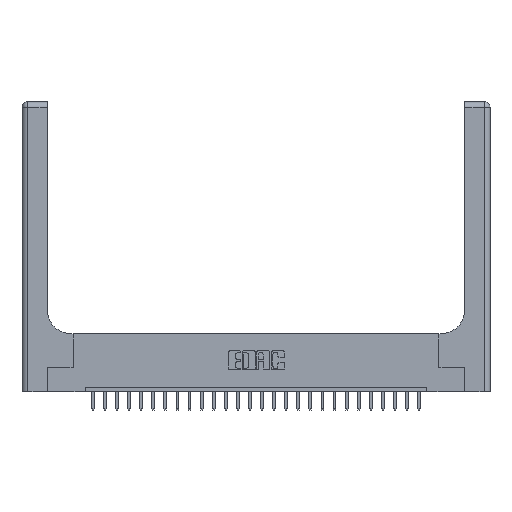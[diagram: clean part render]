
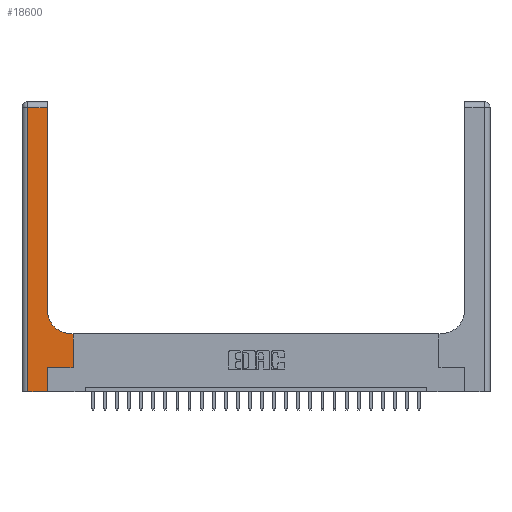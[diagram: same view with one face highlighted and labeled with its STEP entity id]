
A CAD part, top view. The second image highlights one B-rep face of the part: STEP entity #18600.
In plain terms, the highlighted planar face has unit normal (0, 0, 1).
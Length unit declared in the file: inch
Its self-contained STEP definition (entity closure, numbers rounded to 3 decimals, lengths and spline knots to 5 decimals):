
#73 = CARTESIAN_POINT ( 'NONE',  ( 0., 3., 0.37 ) ) ;
#515 = VERTEX_POINT ( 'NONE', #4664 ) ;
#550 = AXIS2_PLACEMENT_3D ( 'NONE', #73, #19193, #1833 ) ;
#741 = CARTESIAN_POINT ( 'NONE',  ( 0., 2.94, 0.37 ) ) ;
#776 = CARTESIAN_POINT ( 'NONE',  ( 0.06, 3., 0.37 ) ) ;
#839 = VECTOR ( 'NONE', #3467, 39.37008 ) ;
#1012 = VERTEX_POINT ( 'NONE', #14244 ) ;
#1243 = ORIENTED_EDGE ( 'NONE', *, *, #19330, .T. ) ;
#1570 = CARTESIAN_POINT ( 'NONE',  ( 0.528, 0.25, 0.37 ) ) ;
#1833 = DIRECTION ( 'NONE',  ( -1., 0., 0. ) ) ;
#2036 = EDGE_CURVE ( 'NONE', #1012, #13675, #19128, .T. ) ;
#2905 = DIRECTION ( 'NONE',  ( 0., -1., 0. ) ) ;
#3044 = DIRECTION ( 'NONE',  ( 0., 1., 0. ) ) ;
#3467 = DIRECTION ( 'NONE',  ( 0., 1., 0. ) ) ;
#3797 = DIRECTION ( 'NONE',  ( 1., 0., 0. ) ) ;
#3840 = ORIENTED_EDGE ( 'NONE', *, *, #20838, .T. ) ;
#3922 = CARTESIAN_POINT ( 'NONE',  ( 0.26, 0.6, 0.37 ) ) ;
#4664 = CARTESIAN_POINT ( 'NONE',  ( 0.06, 2.94, 0.37 ) ) ;
#4860 = VERTEX_POINT ( 'NONE', #6270 ) ;
#4895 = CARTESIAN_POINT ( 'NONE',  ( 0.265, 0., 0.37 ) ) ;
#5770 = DIRECTION ( 'NONE',  ( 0., 0., -1. ) ) ;
#5779 = VERTEX_POINT ( 'NONE', #9205 ) ;
#5790 = EDGE_LOOP ( 'NONE', ( #1243, #3840, #23263, #8727, #20140, #9080, #13010, #18107, #13633 ) ) ;
#6062 = CARTESIAN_POINT ( 'NONE',  ( 0.265, 0.25, 0.37 ) ) ;
#6270 = CARTESIAN_POINT ( 'NONE',  ( 0.06, 0., 0.37 ) ) ;
#7273 = VECTOR ( 'NONE', #23653, 39.37008 ) ;
#7275 = CARTESIAN_POINT ( 'NONE',  ( 0.528, 0.6, 0.37 ) ) ;
#7510 = VERTEX_POINT ( 'NONE', #7275 ) ;
#7710 = VECTOR ( 'NONE', #13552, 39.37008 ) ;
#8296 = CARTESIAN_POINT ( 'NONE',  ( 0.26, 2.94, 0.37 ) ) ;
#8441 = DIRECTION ( 'NONE',  ( -1., 0., 0. ) ) ;
#8727 = ORIENTED_EDGE ( 'NONE', *, *, #12777, .T. ) ;
#9080 = ORIENTED_EDGE ( 'NONE', *, *, #2036, .T. ) ;
#9205 = CARTESIAN_POINT ( 'NONE',  ( 0.26, 0.85, 0.37 ) ) ;
#9413 = FACE_OUTER_BOUND ( 'NONE', #5790, .T. ) ;
#9996 = CARTESIAN_POINT ( 'NONE',  ( 0.51, 0.6, 0.37 ) ) ;
#10021 = LINE ( 'NONE', #15847, #12925 ) ;
#10507 = LINE ( 'NONE', #14680, #18764 ) ;
#11520 = EDGE_CURVE ( 'NONE', #7510, #13034, #19633, .T. ) ;
#11776 = CARTESIAN_POINT ( 'NONE',  ( 0.528, 0.25, 0.37 ) ) ;
#11899 = LINE ( 'NONE', #11776, #7710 ) ;
#12273 = LINE ( 'NONE', #776, #13509 ) ;
#12777 = EDGE_CURVE ( 'NONE', #4860, #14941, #10021, .T. ) ;
#12925 = VECTOR ( 'NONE', #16975, 39.37008 ) ;
#13010 = ORIENTED_EDGE ( 'NONE', *, *, #14116, .T. ) ;
#13034 = VERTEX_POINT ( 'NONE', #9996 ) ;
#13509 = VECTOR ( 'NONE', #2905, 39.37008 ) ;
#13543 = VECTOR ( 'NONE', #8441, 39.37008 ) ;
#13552 = DIRECTION ( 'NONE',  ( 0., 1., 0. ) ) ;
#13611 = EDGE_CURVE ( 'NONE', #14941, #1012, #22964, .T. ) ;
#13633 = ORIENTED_EDGE ( 'NONE', *, *, #16988, .T. ) ;
#13675 = VERTEX_POINT ( 'NONE', #1570 ) ;
#14116 = EDGE_CURVE ( 'NONE', #13675, #7510, #11899, .T. ) ;
#14244 = CARTESIAN_POINT ( 'NONE',  ( 0.265, 0.25, 0.37 ) ) ;
#14680 = CARTESIAN_POINT ( 'NONE',  ( 0.26, 3., 0.37 ) ) ;
#14941 = VERTEX_POINT ( 'NONE', #4895 ) ;
#15847 = CARTESIAN_POINT ( 'NONE',  ( 0., 0., 0.37 ) ) ;
#16975 = DIRECTION ( 'NONE',  ( 1., 0., 0. ) ) ;
#16988 = EDGE_CURVE ( 'NONE', #13034, #5779, #17922, .T. ) ;
#17303 = DIRECTION ( 'NONE',  ( 1., 0., 0. ) ) ;
#17399 = PLANE ( 'NONE',  #550 ) ;
#17922 = CIRCLE ( 'NONE', #19168, 0.25 ) ;
#18107 = ORIENTED_EDGE ( 'NONE', *, *, #11520, .T. ) ;
#18186 = EDGE_CURVE ( 'NONE', #515, #4860, #12273, .T. ) ;
#18600 = ADVANCED_FACE ( 'NONE', ( #9413 ), #17399, .F. ) ;
#18764 = VECTOR ( 'NONE', #3044, 39.37008 ) ;
#19128 = LINE ( 'NONE', #6062, #22414 ) ;
#19168 = AXIS2_PLACEMENT_3D ( 'NONE', #20996, #5770, #17303 ) ;
#19193 = DIRECTION ( 'NONE',  ( 0., 0., -1. ) ) ;
#19330 = EDGE_CURVE ( 'NONE', #5779, #22185, #10507, .T. ) ;
#19633 = LINE ( 'NONE', #3922, #7273 ) ;
#20140 = ORIENTED_EDGE ( 'NONE', *, *, #13611, .T. ) ;
#20705 = CARTESIAN_POINT ( 'NONE',  ( 0.265, 0., 0.37 ) ) ;
#20838 = EDGE_CURVE ( 'NONE', #22185, #515, #24263, .T. ) ;
#20996 = CARTESIAN_POINT ( 'NONE',  ( 0.51, 0.85, 0.37 ) ) ;
#22185 = VERTEX_POINT ( 'NONE', #8296 ) ;
#22414 = VECTOR ( 'NONE', #3797, 39.37008 ) ;
#22964 = LINE ( 'NONE', #20705, #839 ) ;
#23263 = ORIENTED_EDGE ( 'NONE', *, *, #18186, .T. ) ;
#23653 = DIRECTION ( 'NONE',  ( -1., 0., 0. ) ) ;
#24263 = LINE ( 'NONE', #741, #13543 ) ;
